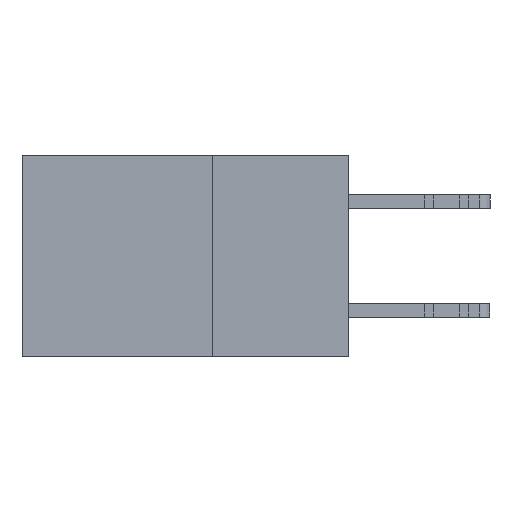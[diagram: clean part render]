
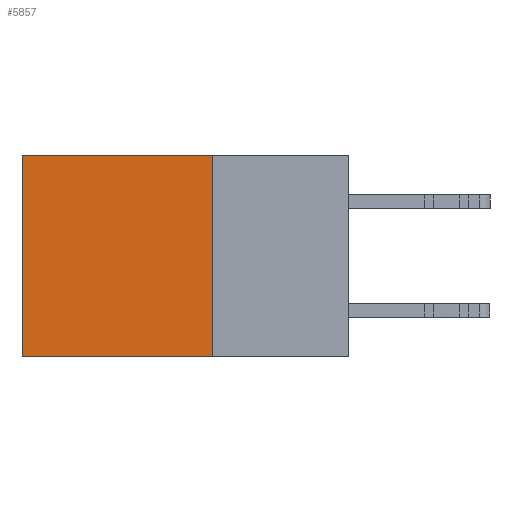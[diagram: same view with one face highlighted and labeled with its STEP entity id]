
A CAD part, left-side view. The second image highlights one B-rep face of the part: STEP entity #5857.
In plain terms, the highlighted planar face has unit normal (-1, 0, 0).
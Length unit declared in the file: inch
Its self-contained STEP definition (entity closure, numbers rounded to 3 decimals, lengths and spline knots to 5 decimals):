
#1189 = VECTOR ( 'NONE', #23734, 39.37008 ) ;
#1262 = CARTESIAN_POINT ( 'NONE',  ( 0.298, 0.25, 0. ) ) ;
#1686 = EDGE_CURVE ( 'NONE', #7564, #12824, #23557, .T. ) ;
#2213 = CARTESIAN_POINT ( 'NONE',  ( 0.298, 0.25, 0. ) ) ;
#2984 = EDGE_LOOP ( 'NONE', ( #4046, #3710, #28558, #21581 ) ) ;
#3710 = ORIENTED_EDGE ( 'NONE', *, *, #14999, .F. ) ;
#4046 = ORIENTED_EDGE ( 'NONE', *, *, #6865, .T. ) ;
#4291 = FACE_OUTER_BOUND ( 'NONE', #2984, .T. ) ;
#5727 = DIRECTION ( 'NONE',  ( 1., 0., 0. ) ) ;
#5857 = ADVANCED_FACE ( 'NONE', ( #4291 ), #12765, .F. ) ;
#6124 = VECTOR ( 'NONE', #23635, 39.37008 ) ;
#6865 = EDGE_CURVE ( 'NONE', #19717, #29832, #13112, .T. ) ;
#7564 = VERTEX_POINT ( 'NONE', #1262 ) ;
#10087 = AXIS2_PLACEMENT_3D ( 'NONE', #19786, #5727, #22212 ) ;
#12765 = PLANE ( 'NONE',  #10087 ) ;
#12824 = VERTEX_POINT ( 'NONE', #25273 ) ;
#13112 = LINE ( 'NONE', #28439, #1189 ) ;
#13793 = CARTESIAN_POINT ( 'NONE',  ( 0.298, 0.6, -0.37 ) ) ;
#14127 = CARTESIAN_POINT ( 'NONE',  ( 0.298, 0.25, -0.37 ) ) ;
#14999 = EDGE_CURVE ( 'NONE', #12824, #29832, #17142, .T. ) ;
#17142 = LINE ( 'NONE', #14127, #6124 ) ;
#19141 = CARTESIAN_POINT ( 'NONE',  ( 0.298, 0.6, 0. ) ) ;
#19717 = VERTEX_POINT ( 'NONE', #19141 ) ;
#19786 = CARTESIAN_POINT ( 'NONE',  ( 0.298, 0.25, 0. ) ) ;
#20134 = LINE ( 'NONE', #2213, #24995 ) ;
#21094 = DIRECTION ( 'NONE',  ( 0., 1., 0. ) ) ;
#21581 = ORIENTED_EDGE ( 'NONE', *, *, #27559, .T. ) ;
#22212 = DIRECTION ( 'NONE',  ( 0., 0., -1. ) ) ;
#23557 = LINE ( 'NONE', #28488, #28311 ) ;
#23635 = DIRECTION ( 'NONE',  ( 0., 1., 0. ) ) ;
#23734 = DIRECTION ( 'NONE',  ( 0., 0., -1. ) ) ;
#24995 = VECTOR ( 'NONE', #21094, 39.37008 ) ;
#25273 = CARTESIAN_POINT ( 'NONE',  ( 0.298, 0.25, -0.37 ) ) ;
#27559 = EDGE_CURVE ( 'NONE', #7564, #19717, #20134, .T. ) ;
#28311 = VECTOR ( 'NONE', #28562, 39.37008 ) ;
#28439 = CARTESIAN_POINT ( 'NONE',  ( 0.298, 0.6, 0. ) ) ;
#28488 = CARTESIAN_POINT ( 'NONE',  ( 0.298, 0.25, 0. ) ) ;
#28558 = ORIENTED_EDGE ( 'NONE', *, *, #1686, .F. ) ;
#28562 = DIRECTION ( 'NONE',  ( 0., 0., -1. ) ) ;
#29832 = VERTEX_POINT ( 'NONE', #13793 ) ;
